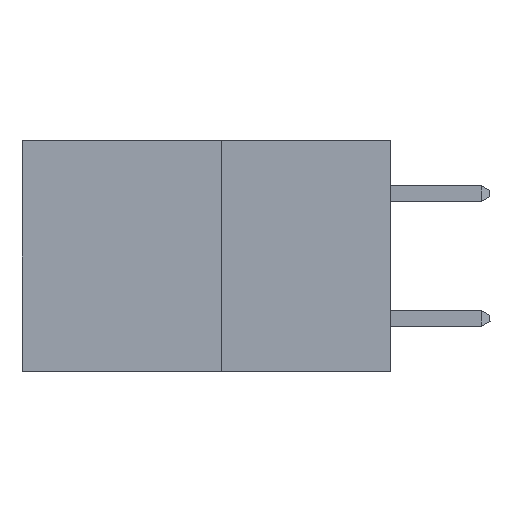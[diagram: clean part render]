
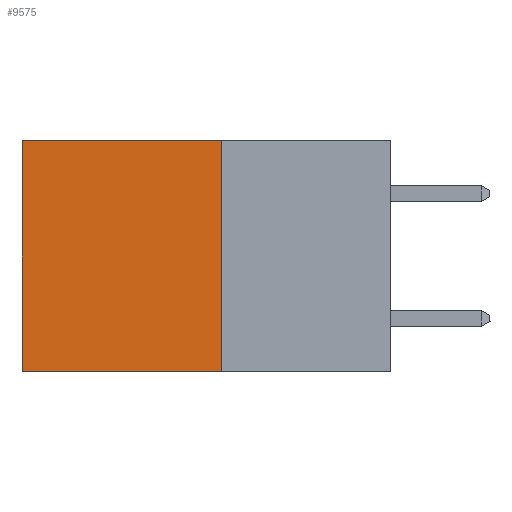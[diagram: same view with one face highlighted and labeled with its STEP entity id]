
A CAD part, left-side view. The second image highlights one B-rep face of the part: STEP entity #9575.
In plain terms, the highlighted planar face has unit normal (-1, 0, 0).
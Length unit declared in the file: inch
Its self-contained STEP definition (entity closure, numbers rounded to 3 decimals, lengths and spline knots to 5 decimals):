
#351 = VECTOR ( 'NONE', #7791, 39.37008 ) ;
#1908 = PLANE ( 'NONE',  #11537 ) ;
#2029 = CARTESIAN_POINT ( 'NONE',  ( 0.277, 0.59, -0.37 ) ) ;
#2209 = LINE ( 'NONE', #2029, #19251 ) ;
#2420 = DIRECTION ( 'NONE',  ( 0., 1., 0. ) ) ;
#2888 = DIRECTION ( 'NONE',  ( 0., 1., 0. ) ) ;
#4524 = ORIENTED_EDGE ( 'NONE', *, *, #11356, .T. ) ;
#5405 = LINE ( 'NONE', #21283, #351 ) ;
#6664 = CARTESIAN_POINT ( 'NONE',  ( 0.277, 0.27, 0. ) ) ;
#7045 = DIRECTION ( 'NONE',  ( 1., 0., 0. ) ) ;
#7791 = DIRECTION ( 'NONE',  ( 0., 0., -1. ) ) ;
#9575 = ADVANCED_FACE ( 'NONE', ( #20768 ), #1908, .F. ) ;
#11356 = EDGE_CURVE ( 'NONE', #21790, #12277, #12541, .T. ) ;
#11537 = AXIS2_PLACEMENT_3D ( 'NONE', #17278, #7045, #18960 ) ;
#12277 = VERTEX_POINT ( 'NONE', #14985 ) ;
#12541 = LINE ( 'NONE', #14848, #20956 ) ;
#13021 = VERTEX_POINT ( 'NONE', #19954 ) ;
#13161 = CARTESIAN_POINT ( 'NONE',  ( 0.277, 0.59, -0.37 ) ) ;
#13236 = LINE ( 'NONE', #19473, #21635 ) ;
#14138 = EDGE_LOOP ( 'NONE', ( #17930, #15641, #17267, #4524 ) ) ;
#14617 = EDGE_CURVE ( 'NONE', #12277, #19065, #2209, .T. ) ;
#14848 = CARTESIAN_POINT ( 'NONE',  ( 0.277, 0.27, 0. ) ) ;
#14985 = CARTESIAN_POINT ( 'NONE',  ( 0.277, 0.59, 0. ) ) ;
#15641 = ORIENTED_EDGE ( 'NONE', *, *, #17629, .F. ) ;
#17267 = ORIENTED_EDGE ( 'NONE', *, *, #18364, .F. ) ;
#17278 = CARTESIAN_POINT ( 'NONE',  ( 0.277, 0.27, -0.37 ) ) ;
#17400 = DIRECTION ( 'NONE',  ( 0., 0., -1. ) ) ;
#17629 = EDGE_CURVE ( 'NONE', #13021, #19065, #13236, .T. ) ;
#17930 = ORIENTED_EDGE ( 'NONE', *, *, #14617, .T. ) ;
#18364 = EDGE_CURVE ( 'NONE', #21790, #13021, #5405, .T. ) ;
#18960 = DIRECTION ( 'NONE',  ( 0., 0., -1. ) ) ;
#19065 = VERTEX_POINT ( 'NONE', #13161 ) ;
#19251 = VECTOR ( 'NONE', #17400, 39.37008 ) ;
#19473 = CARTESIAN_POINT ( 'NONE',  ( 0.277, 0.27, -0.37 ) ) ;
#19954 = CARTESIAN_POINT ( 'NONE',  ( 0.277, 0.27, -0.37 ) ) ;
#20768 = FACE_OUTER_BOUND ( 'NONE', #14138, .T. ) ;
#20956 = VECTOR ( 'NONE', #2888, 39.37008 ) ;
#21283 = CARTESIAN_POINT ( 'NONE',  ( 0.277, 0.27, -0.37 ) ) ;
#21635 = VECTOR ( 'NONE', #2420, 39.37008 ) ;
#21790 = VERTEX_POINT ( 'NONE', #6664 ) ;
